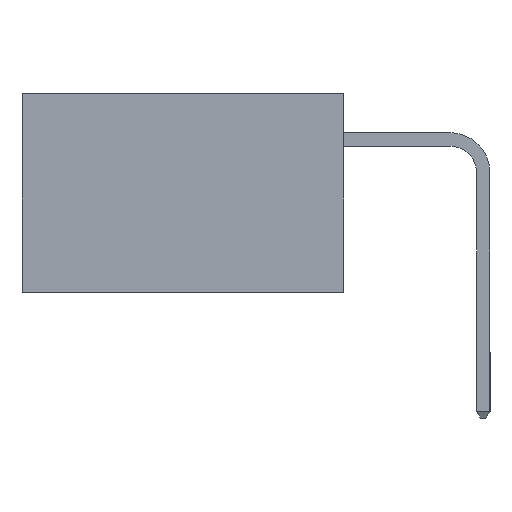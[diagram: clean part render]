
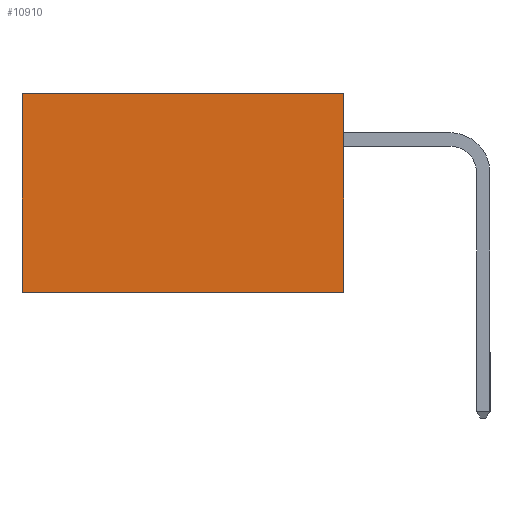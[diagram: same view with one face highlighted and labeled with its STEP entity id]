
A CAD part, left-side view. The second image highlights one B-rep face of the part: STEP entity #10910.
In plain terms, the highlighted planar face has unit normal (-1, 0, 0).
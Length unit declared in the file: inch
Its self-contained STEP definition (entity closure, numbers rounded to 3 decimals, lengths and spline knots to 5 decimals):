
#243 = VERTEX_POINT ( 'NONE', #7000 ) ;
#519 = DIRECTION ( 'NONE',  ( 0., 1., 0. ) ) ;
#1559 = CARTESIAN_POINT ( 'NONE',  ( 0.298, 0., -0.37 ) ) ;
#1861 = VERTEX_POINT ( 'NONE', #6251 ) ;
#2077 = EDGE_CURVE ( 'NONE', #1861, #12902, #3303, .T. ) ;
#2868 = CARTESIAN_POINT ( 'NONE',  ( 0.298, 0.6, 0. ) ) ;
#2973 = PLANE ( 'NONE',  #14399 ) ;
#3303 = LINE ( 'NONE', #11527, #14035 ) ;
#4224 = VECTOR ( 'NONE', #13794, 39.37008 ) ;
#4847 = DIRECTION ( 'NONE',  ( 0., 1., 0. ) ) ;
#4919 = VECTOR ( 'NONE', #4847, 39.37008 ) ;
#4951 = ORIENTED_EDGE ( 'NONE', *, *, #2077, .F. ) ;
#5006 = DIRECTION ( 'NONE',  ( 0., 0., -1. ) ) ;
#5831 = VERTEX_POINT ( 'NONE', #2868 ) ;
#5935 = VECTOR ( 'NONE', #519, 39.37008 ) ;
#6244 = DIRECTION ( 'NONE',  ( 1., 0., 0. ) ) ;
#6251 = CARTESIAN_POINT ( 'NONE',  ( 0.298, 0., 0. ) ) ;
#7000 = CARTESIAN_POINT ( 'NONE',  ( 0.298, 0.6, -0.37 ) ) ;
#7617 = CARTESIAN_POINT ( 'NONE',  ( 0.298, 0., -0.37 ) ) ;
#9521 = EDGE_LOOP ( 'NONE', ( #12733, #19719, #4951, #11781 ) ) ;
#10304 = LINE ( 'NONE', #1559, #4919 ) ;
#10910 = ADVANCED_FACE ( 'NONE', ( #16950 ), #2973, .F. ) ;
#11527 = CARTESIAN_POINT ( 'NONE',  ( 0.298, 0., 0. ) ) ;
#11781 = ORIENTED_EDGE ( 'NONE', *, *, #18678, .T. ) ;
#12733 = ORIENTED_EDGE ( 'NONE', *, *, #16646, .T. ) ;
#12817 = DIRECTION ( 'NONE',  ( 0., 0., -1. ) ) ;
#12841 = LINE ( 'NONE', #15476, #5935 ) ;
#12902 = VERTEX_POINT ( 'NONE', #7617 ) ;
#13794 = DIRECTION ( 'NONE',  ( 0., 0., -1. ) ) ;
#14035 = VECTOR ( 'NONE', #5006, 39.37008 ) ;
#14310 = CARTESIAN_POINT ( 'NONE',  ( 0.298, 0., 0. ) ) ;
#14399 = AXIS2_PLACEMENT_3D ( 'NONE', #14310, #6244, #12817 ) ;
#15476 = CARTESIAN_POINT ( 'NONE',  ( 0.298, 0., 0. ) ) ;
#15571 = CARTESIAN_POINT ( 'NONE',  ( 0.298, 0.6, 0. ) ) ;
#16646 = EDGE_CURVE ( 'NONE', #5831, #243, #18227, .T. ) ;
#16950 = FACE_OUTER_BOUND ( 'NONE', #9521, .T. ) ;
#17975 = EDGE_CURVE ( 'NONE', #12902, #243, #10304, .T. ) ;
#18227 = LINE ( 'NONE', #15571, #4224 ) ;
#18678 = EDGE_CURVE ( 'NONE', #1861, #5831, #12841, .T. ) ;
#19719 = ORIENTED_EDGE ( 'NONE', *, *, #17975, .F. ) ;
